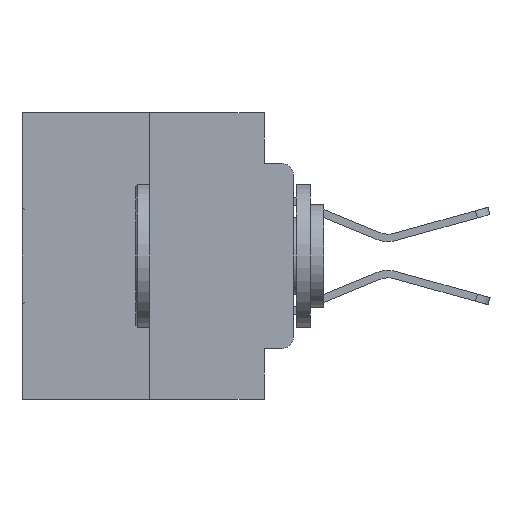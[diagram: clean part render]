
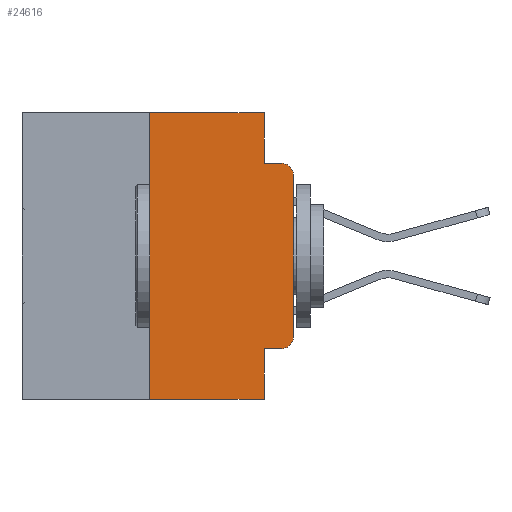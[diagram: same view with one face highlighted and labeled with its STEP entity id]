
A CAD part, left-side view. The second image highlights one B-rep face of the part: STEP entity #24616.
In plain terms, the highlighted planar face has unit normal (-1, 0, 0).
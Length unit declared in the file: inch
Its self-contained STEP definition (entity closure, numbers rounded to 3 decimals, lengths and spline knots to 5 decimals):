
#292 = AXIS2_PLACEMENT_3D ( 'NONE', #17863, #8004, #25581 ) ;
#470 = DIRECTION ( 'NONE',  ( 0., 0., -1. ) ) ;
#1083 = DIRECTION ( 'NONE',  ( 0., 0., 1. ) ) ;
#2296 = ORIENTED_EDGE ( 'NONE', *, *, #8938, .F. ) ;
#2612 = FACE_OUTER_BOUND ( 'NONE', #9338, .T. ) ;
#2671 = CARTESIAN_POINT ( 'NONE',  ( 0., 0.051, -0.0885 ) ) ;
#3052 = CARTESIAN_POINT ( 'NONE',  ( 0., 0.051, 0. ) ) ;
#3255 = VERTEX_POINT ( 'NONE', #22945 ) ;
#3480 = AXIS2_PLACEMENT_3D ( 'NONE', #17681, #27700, #470 ) ;
#3657 = DIRECTION ( 'NONE',  ( 0., 0., 1. ) ) ;
#4012 = CIRCLE ( 'NONE', #8710, 0.02 ) ;
#4060 = VECTOR ( 'NONE', #1083, 39.37008 ) ;
#4917 = DIRECTION ( 'NONE',  ( 0., -1., 0. ) ) ;
#5113 = VECTOR ( 'NONE', #8005, 39.37008 ) ;
#5165 = ORIENTED_EDGE ( 'NONE', *, *, #29124, .F. ) ;
#6202 = VERTEX_POINT ( 'NONE', #15120 ) ;
#6298 = VERTEX_POINT ( 'NONE', #11001 ) ;
#6776 = EDGE_CURVE ( 'NONE', #3255, #28979, #23281, .T. ) ;
#8004 = DIRECTION ( 'NONE',  ( 1., 0., 0. ) ) ;
#8005 = DIRECTION ( 'NONE',  ( 0., -1., 0. ) ) ;
#8042 = DIRECTION ( 'NONE',  ( 0., 0., -1. ) ) ;
#8413 = ORIENTED_EDGE ( 'NONE', *, *, #15292, .F. ) ;
#8610 = VERTEX_POINT ( 'NONE', #24788 ) ;
#8710 = AXIS2_PLACEMENT_3D ( 'NONE', #20161, #25239, #22953 ) ;
#8938 = EDGE_CURVE ( 'NONE', #16735, #28513, #27218, .T. ) ;
#9057 = VECTOR ( 'NONE', #14898, 39.37008 ) ;
#9338 = EDGE_LOOP ( 'NONE', ( #13103, #9815, #2296, #10622, #17637, #5165, #20784, #8413, #28938, #11962 ) ) ;
#9365 = VECTOR ( 'NONE', #11510, 39.37008 ) ;
#9815 = ORIENTED_EDGE ( 'NONE', *, *, #28502, .T. ) ;
#10123 = CARTESIAN_POINT ( 'NONE',  ( 0., 0.051, -0.0885 ) ) ;
#10622 = ORIENTED_EDGE ( 'NONE', *, *, #24194, .F. ) ;
#11001 = CARTESIAN_POINT ( 'NONE',  ( 0., 0.02, -0.4115 ) ) ;
#11262 = VECTOR ( 'NONE', #8042, 39.37008 ) ;
#11281 = EDGE_CURVE ( 'NONE', #6202, #19772, #16445, .T. ) ;
#11510 = DIRECTION ( 'NONE',  ( 0., 0., -1. ) ) ;
#11962 = ORIENTED_EDGE ( 'NONE', *, *, #28461, .T. ) ;
#12299 = CARTESIAN_POINT ( 'NONE',  ( 0., 0.051, -0.4115 ) ) ;
#12410 = VECTOR ( 'NONE', #30816, 39.37008 ) ;
#13103 = ORIENTED_EDGE ( 'NONE', *, *, #11281, .T. ) ;
#14898 = DIRECTION ( 'NONE',  ( 0., -1., 0. ) ) ;
#15120 = CARTESIAN_POINT ( 'NONE',  ( 0., 0., -0.3915 ) ) ;
#15292 = EDGE_CURVE ( 'NONE', #8610, #15941, #31696, .T. ) ;
#15551 = EDGE_CURVE ( 'NONE', #8610, #6298, #17553, .T. ) ;
#15941 = VERTEX_POINT ( 'NONE', #27647 ) ;
#15996 = LINE ( 'NONE', #16324, #4060 ) ;
#16324 = CARTESIAN_POINT ( 'NONE',  ( 0., 0.25, 0. ) ) ;
#16445 = LINE ( 'NONE', #28769, #19822 ) ;
#16735 = VERTEX_POINT ( 'NONE', #2671 ) ;
#16803 = CARTESIAN_POINT ( 'NONE',  ( 0., 0.473, -0.5 ) ) ;
#16912 = CARTESIAN_POINT ( 'NONE',  ( 0., 0.051, 0. ) ) ;
#17368 = VERTEX_POINT ( 'NONE', #29633 ) ;
#17553 = LINE ( 'NONE', #12299, #26690 ) ;
#17637 = ORIENTED_EDGE ( 'NONE', *, *, #6776, .F. ) ;
#17681 = CARTESIAN_POINT ( 'NONE',  ( 0., 0.02, -0.1085 ) ) ;
#17723 = CARTESIAN_POINT ( 'NONE',  ( 0., 0., -0.1085 ) ) ;
#17863 = CARTESIAN_POINT ( 'NONE',  ( 0., 0.473, 0. ) ) ;
#18166 = CARTESIAN_POINT ( 'NONE',  ( 0., 0.02, -0.0885 ) ) ;
#19772 = VERTEX_POINT ( 'NONE', #17723 ) ;
#19822 = VECTOR ( 'NONE', #3657, 39.37008 ) ;
#20161 = CARTESIAN_POINT ( 'NONE',  ( 0., 0.02, -0.3915 ) ) ;
#20784 = ORIENTED_EDGE ( 'NONE', *, *, #27266, .T. ) ;
#21296 = LINE ( 'NONE', #16803, #12410 ) ;
#22634 = PLANE ( 'NONE',  #292 ) ;
#22945 = CARTESIAN_POINT ( 'NONE',  ( 0., 0.25, 0. ) ) ;
#22953 = DIRECTION ( 'NONE',  ( 0., 0., -1. ) ) ;
#23004 = CARTESIAN_POINT ( 'NONE',  ( 0., 0.051, 0. ) ) ;
#23281 = LINE ( 'NONE', #23444, #5113 ) ;
#23444 = CARTESIAN_POINT ( 'NONE',  ( 0., 0.473, 0. ) ) ;
#23480 = LINE ( 'NONE', #23004, #11262 ) ;
#24194 = EDGE_CURVE ( 'NONE', #28979, #16735, #23480, .T. ) ;
#24439 = CIRCLE ( 'NONE', #3480, 0.02 ) ;
#24616 = ADVANCED_FACE ( 'NONE', ( #2612 ), #22634, .F. ) ;
#24788 = CARTESIAN_POINT ( 'NONE',  ( 0., 0.051, -0.4115 ) ) ;
#25239 = DIRECTION ( 'NONE',  ( -1., 0., 0. ) ) ;
#25581 = DIRECTION ( 'NONE',  ( 0., 0., -1. ) ) ;
#26690 = VECTOR ( 'NONE', #4917, 39.37008 ) ;
#27218 = LINE ( 'NONE', #10123, #9057 ) ;
#27266 = EDGE_CURVE ( 'NONE', #17368, #15941, #21296, .T. ) ;
#27647 = CARTESIAN_POINT ( 'NONE',  ( 0., 0.051, -0.5 ) ) ;
#27700 = DIRECTION ( 'NONE',  ( -1., 0., 0. ) ) ;
#28461 = EDGE_CURVE ( 'NONE', #6298, #6202, #4012, .T. ) ;
#28502 = EDGE_CURVE ( 'NONE', #19772, #28513, #24439, .T. ) ;
#28513 = VERTEX_POINT ( 'NONE', #18166 ) ;
#28769 = CARTESIAN_POINT ( 'NONE',  ( 0., 0., 0. ) ) ;
#28938 = ORIENTED_EDGE ( 'NONE', *, *, #15551, .T. ) ;
#28979 = VERTEX_POINT ( 'NONE', #3052 ) ;
#29124 = EDGE_CURVE ( 'NONE', #17368, #3255, #15996, .T. ) ;
#29633 = CARTESIAN_POINT ( 'NONE',  ( 0., 0.25, -0.5 ) ) ;
#30816 = DIRECTION ( 'NONE',  ( 0., -1., 0. ) ) ;
#31696 = LINE ( 'NONE', #16912, #9365 ) ;
